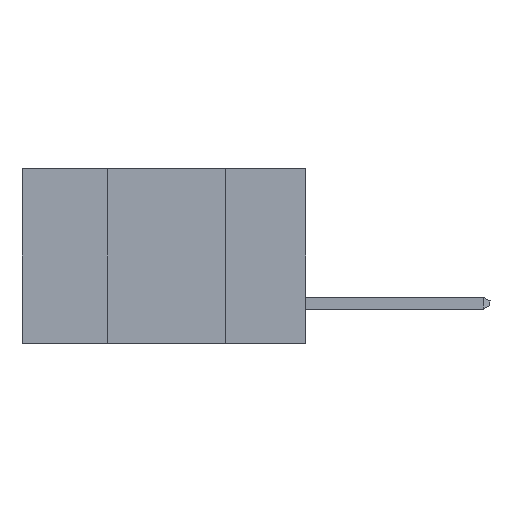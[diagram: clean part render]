
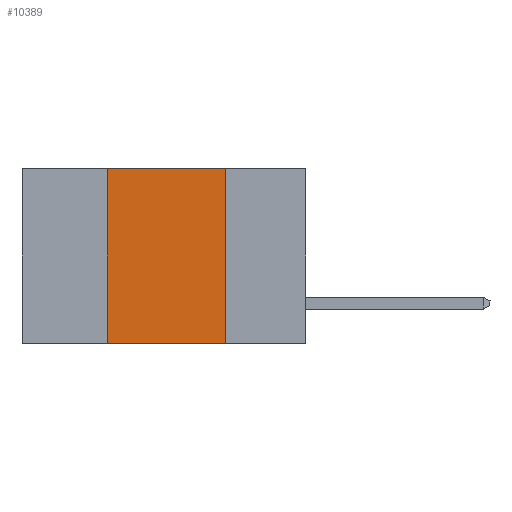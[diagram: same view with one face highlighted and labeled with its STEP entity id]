
A CAD part, left-side view. The second image highlights one B-rep face of the part: STEP entity #10389.
In plain terms, the highlighted planar face has unit normal (-1, 0, 0).
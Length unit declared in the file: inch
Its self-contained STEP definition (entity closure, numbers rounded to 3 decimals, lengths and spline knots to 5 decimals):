
#655 = DIRECTION ( 'NONE',  ( 0., 0., -1. ) ) ;
#661 = CARTESIAN_POINT ( 'NONE',  ( 0., 0.17, -0.37 ) ) ;
#1166 = VECTOR ( 'NONE', #24865, 39.37008 ) ;
#1532 = VECTOR ( 'NONE', #3400, 39.37008 ) ;
#2891 = PLANE ( 'NONE',  #3501 ) ;
#3369 = ORIENTED_EDGE ( 'NONE', *, *, #15525, .T. ) ;
#3400 = DIRECTION ( 'NONE',  ( 0., -1., 0. ) ) ;
#3501 = AXIS2_PLACEMENT_3D ( 'NONE', #8638, #6953, #655 ) ;
#4977 = CARTESIAN_POINT ( 'NONE',  ( 0., 0.42, -0.37 ) ) ;
#5034 = EDGE_CURVE ( 'NONE', #15579, #20911, #18707, .T. ) ;
#5998 = ORIENTED_EDGE ( 'NONE', *, *, #14307, .F. ) ;
#6953 = DIRECTION ( 'NONE',  ( 1., 0., 0. ) ) ;
#7003 = CARTESIAN_POINT ( 'NONE',  ( 0., 0.42, 0. ) ) ;
#7226 = LINE ( 'NONE', #17024, #1166 ) ;
#7541 = LINE ( 'NONE', #23471, #14216 ) ;
#8638 = CARTESIAN_POINT ( 'NONE',  ( 0., 0.6, 0. ) ) ;
#9171 = FACE_OUTER_BOUND ( 'NONE', #19188, .T. ) ;
#9202 = ORIENTED_EDGE ( 'NONE', *, *, #21194, .F. ) ;
#10389 = ADVANCED_FACE ( 'NONE', ( #9171 ), #2891, .F. ) ;
#10399 = VERTEX_POINT ( 'NONE', #4977 ) ;
#11247 = CARTESIAN_POINT ( 'NONE',  ( 0., 0.6, 0. ) ) ;
#13116 = ORIENTED_EDGE ( 'NONE', *, *, #5034, .F. ) ;
#14216 = VECTOR ( 'NONE', #19562, 39.37008 ) ;
#14307 = EDGE_CURVE ( 'NONE', #21389, #15579, #15274, .T. ) ;
#15274 = LINE ( 'NONE', #11247, #1532 ) ;
#15525 = EDGE_CURVE ( 'NONE', #10399, #20911, #7226, .T. ) ;
#15579 = VERTEX_POINT ( 'NONE', #22765 ) ;
#17024 = CARTESIAN_POINT ( 'NONE',  ( 0., 0.6, -0.37 ) ) ;
#18707 = LINE ( 'NONE', #661, #25143 ) ;
#19188 = EDGE_LOOP ( 'NONE', ( #13116, #5998, #9202, #3369 ) ) ;
#19562 = DIRECTION ( 'NONE',  ( 0., 0., 1. ) ) ;
#20473 = CARTESIAN_POINT ( 'NONE',  ( 0., 0.17, -0.37 ) ) ;
#20911 = VERTEX_POINT ( 'NONE', #20473 ) ;
#21194 = EDGE_CURVE ( 'NONE', #10399, #21389, #7541, .T. ) ;
#21389 = VERTEX_POINT ( 'NONE', #7003 ) ;
#22751 = DIRECTION ( 'NONE',  ( 0., 0., -1. ) ) ;
#22765 = CARTESIAN_POINT ( 'NONE',  ( 0., 0.17, 0. ) ) ;
#23471 = CARTESIAN_POINT ( 'NONE',  ( 0., 0.42, -0.37 ) ) ;
#24865 = DIRECTION ( 'NONE',  ( 0., -1., 0. ) ) ;
#25143 = VECTOR ( 'NONE', #22751, 39.37008 ) ;
